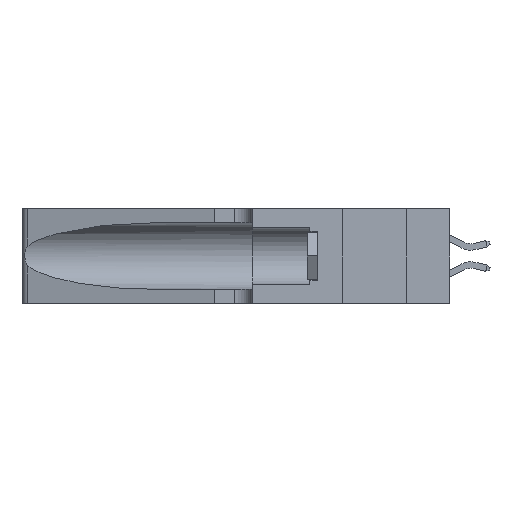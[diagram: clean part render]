
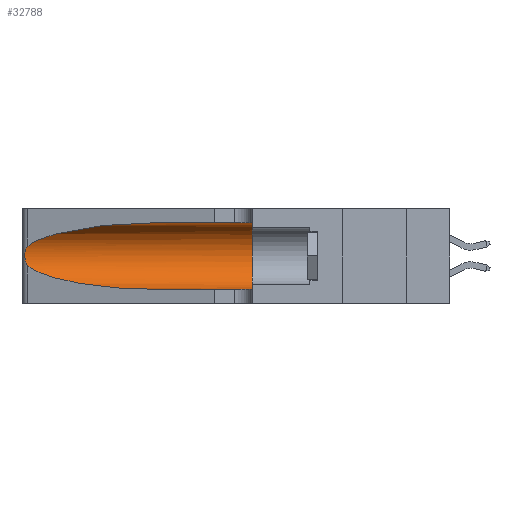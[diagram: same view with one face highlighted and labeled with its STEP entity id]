
A CAD part, left-side view. The second image highlights one B-rep face of the part: STEP entity #32788.
In plain terms, the highlighted cylindrical face has radius 3.308 mm (diameter 6.617 mm), a partial arc.
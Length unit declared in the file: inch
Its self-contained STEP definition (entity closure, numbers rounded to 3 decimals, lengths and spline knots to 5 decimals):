
#671 = ORIENTED_EDGE ( 'NONE', *, *, #21049, .T. ) ;
#1794 = CARTESIAN_POINT ( 'NONE',  ( 0.1305, 0.72297, 0.05475 ) ) ;
#2954 = CARTESIAN_POINT ( 'NONE',  ( 0.26018, 1.23835, 0.19895 ) ) ;
#2966 = CARTESIAN_POINT ( 'NONE',  ( 0.1305, 1.61858, 0.185 ) ) ;
#3782 = CARTESIAN_POINT ( 'NONE',  ( 0.25487, 1.22718, 0.14631 ) ) ;
#3834 = VERTEX_POINT ( 'NONE', #4356 ) ;
#4356 = CARTESIAN_POINT ( 'NONE',  ( 0.1305, 0.35, 0.31525 ) ) ;
#4379 = CYLINDRICAL_SURFACE ( 'NONE', #37900, 0.13025 ) ;
#5687 = EDGE_CURVE ( 'NONE', #27841, #3834, #21451, .T. ) ;
#5817 = B_SPLINE_CURVE_WITH_KNOTS ( 'NONE', 3,
 ( #29740, #32772, #17979, #38729, #20982, #2954, #23940, #6003, #26890, #9125, #29866, #12142, #32902, #15116 ),
 .UNSPECIFIED., .F., .F.,
 ( 4, 2, 2, 2, 2, 2, 4 ),
 ( 0., 0.00027, 0.00053, 0.00107, 0.0016, 0.00187, 0.00214 ),
 .UNSPECIFIED. ) ;
#5873 = EDGE_LOOP ( 'NONE', ( #17829, #671, #11214, #19600, #30724, #11286 ) ) ;
#6003 = CARTESIAN_POINT ( 'NONE',  ( 0.26075, 1.23896, 0.178 ) ) ;
#7468 = CARTESIAN_POINT ( 'NONE',  ( 0.1305, 0.35, 0.185 ) ) ;
#8221 = CARTESIAN_POINT ( 'NONE',  ( 0.1305, 1.61858, 0.05475 ) ) ;
#8584 = CARTESIAN_POINT ( 'NONE',  ( 0.1305, 0.72297, 0.31525 ) ) ;
#9125 = CARTESIAN_POINT ( 'NONE',  ( 0.25856, 1.23593, 0.16098 ) ) ;
#9134 = DIRECTION ( 'NONE',  ( 0., -1., 0. ) ) ;
#9141 = VERTEX_POINT ( 'NONE', #17843 ) ;
#9515 = CIRCLE ( 'NONE', #35648, 0.13025 ) ;
#10571 = DIRECTION ( 'NONE',  ( 0., 0., 1. ) ) ;
#11214 = ORIENTED_EDGE ( 'NONE', *, *, #12535, .T. ) ;
#11286 = ORIENTED_EDGE ( 'NONE', *, *, #5687, .F. ) ;
#12142 = CARTESIAN_POINT ( 'NONE',  ( 0.25639, 1.23186, 0.15144 ) ) ;
#12363 = VERTEX_POINT ( 'NONE', #3782 ) ;
#12535 = EDGE_CURVE ( 'NONE', #12363, #15259, #36829, .T. ) ;
#13622 = CARTESIAN_POINT ( 'NONE',  ( 0.25487, 1.22718, 0.22369 ) ) ;
#15116 = CARTESIAN_POINT ( 'NONE',  ( 0.25487, 1.22718, 0.14631 ) ) ;
#15259 = VERTEX_POINT ( 'NONE', #37474 ) ;
#16086 = CARTESIAN_POINT ( 'NONE',  ( 0.1305, 0.35, 0.05475 ) ) ;
#17829 = ORIENTED_EDGE ( 'NONE', *, *, #18453, .T. ) ;
#17843 = CARTESIAN_POINT ( 'NONE',  ( 0.25487, 1.22718, 0.22369 ) ) ;
#17979 = CARTESIAN_POINT ( 'NONE',  ( 0.25639, 1.23184, 0.21858 ) ) ;
#18453 = EDGE_CURVE ( 'NONE', #27841, #9141, #32702, .T. ) ;
#19376 = EDGE_CURVE ( 'NONE', #3834, #19946, #9515, .T. ) ;
#19600 = ORIENTED_EDGE ( 'NONE', *, *, #25220, .T. ) ;
#19844 = CARTESIAN_POINT ( 'NONE',  ( 0.18966, 0.96281, 0.05475 ) ) ;
#19946 = VERTEX_POINT ( 'NONE', #16086 ) ;
#20522 = VECTOR ( 'NONE', #21313, 39.37008 ) ;
#20982 = CARTESIAN_POINT ( 'NONE',  ( 0.25854, 1.2359, 0.20912 ) ) ;
#21049 = EDGE_CURVE ( 'NONE', #9141, #12363, #5817, .T. ) ;
#21313 = DIRECTION ( 'NONE',  ( 0., -1., 0. ) ) ;
#21451 = LINE ( 'NONE', #27339, #20522 ) ;
#22460 = CARTESIAN_POINT ( 'NONE',  ( 0.18966, 0.96281, 0.31525 ) ) ;
#23940 = CARTESIAN_POINT ( 'NONE',  ( 0.26075, 1.23896, 0.19203 ) ) ;
#25220 = EDGE_CURVE ( 'NONE', #15259, #19946, #31287, .T. ) ;
#25418 = CARTESIAN_POINT ( 'NONE',  ( 0.1305, 0.72297, 0.31525 ) ) ;
#25659 = CARTESIAN_POINT ( 'NONE',  ( 0.2373, 1.15595, 0.08982 ) ) ;
#26890 = CARTESIAN_POINT ( 'NONE',  ( 0.26017, 1.23833, 0.17102 ) ) ;
#27339 = CARTESIAN_POINT ( 'NONE',  ( 0.1305, 1.61858, 0.31525 ) ) ;
#27841 = VERTEX_POINT ( 'NONE', #8584 ) ;
#28304 = DIRECTION ( 'NONE',  ( 0., 1., 0. ) ) ;
#29740 = CARTESIAN_POINT ( 'NONE',  ( 0.25487, 1.22718, 0.22369 ) ) ;
#29866 = CARTESIAN_POINT ( 'NONE',  ( 0.25789, 1.23486, 0.15765 ) ) ;
#29870 = DIRECTION ( 'NONE',  ( 0., 0., -1. ) ) ;
#30724 = ORIENTED_EDGE ( 'NONE', *, *, #19376, .F. ) ;
#31287 = LINE ( 'NONE', #8221, #37331 ) ;
#31392 = CARTESIAN_POINT ( 'NONE',  ( 0.2373, 1.15595, 0.28018 ) ) ;
#32022 = DIRECTION ( 'NONE',  ( 0., -1., 0. ) ) ;
#32702 =( BOUNDED_CURVE ( )  B_SPLINE_CURVE ( 3, ( #25418, #22460, #31392, #13622 ),
 .UNSPECIFIED., .F., .F. ) 
 B_SPLINE_CURVE_WITH_KNOTS ( ( 4, 4 ),
 ( 1.5708, 2.84003 ),
 .UNSPECIFIED. ) 
 CURVE ( )  GEOMETRIC_REPRESENTATION_ITEM ( )  RATIONAL_B_SPLINE_CURVE ( ( 1., 0.87, 0.87, 1. ) ) 
 REPRESENTATION_ITEM ( '' )  );
#32772 = CARTESIAN_POINT ( 'NONE',  ( 0.25555, 1.22994, 0.2215 ) ) ;
#32788 = ADVANCED_FACE ( 'NONE', ( #37081 ), #4379, .F. ) ;
#32902 = CARTESIAN_POINT ( 'NONE',  ( 0.25555, 1.22993, 0.14849 ) ) ;
#34629 = CARTESIAN_POINT ( 'NONE',  ( 0.25487, 1.22718, 0.14631 ) ) ;
#35648 = AXIS2_PLACEMENT_3D ( 'NONE', #7468, #28304, #10571 ) ;
#36829 =( BOUNDED_CURVE ( )  B_SPLINE_CURVE ( 3, ( #34629, #25659, #19844, #1794 ),
 .UNSPECIFIED., .F., .F. ) 
 B_SPLINE_CURVE_WITH_KNOTS ( ( 4, 4 ),
 ( 3.44316, 4.71239 ),
 .UNSPECIFIED. ) 
 CURVE ( )  GEOMETRIC_REPRESENTATION_ITEM ( )  RATIONAL_B_SPLINE_CURVE ( ( 1., 0.87, 0.87, 1. ) ) 
 REPRESENTATION_ITEM ( '' )  );
#37081 = FACE_OUTER_BOUND ( 'NONE', #5873, .T. ) ;
#37331 = VECTOR ( 'NONE', #32022, 39.37008 ) ;
#37474 = CARTESIAN_POINT ( 'NONE',  ( 0.1305, 0.72297, 0.05475 ) ) ;
#37900 = AXIS2_PLACEMENT_3D ( 'NONE', #2966, #9134, #29870 ) ;
#38729 = CARTESIAN_POINT ( 'NONE',  ( 0.25787, 1.23484, 0.2124 ) ) ;
